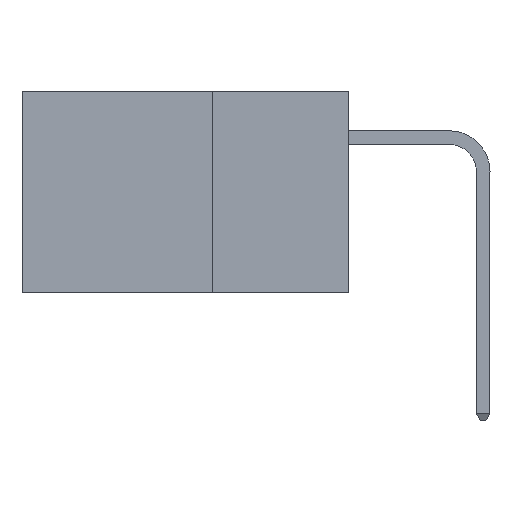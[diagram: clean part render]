
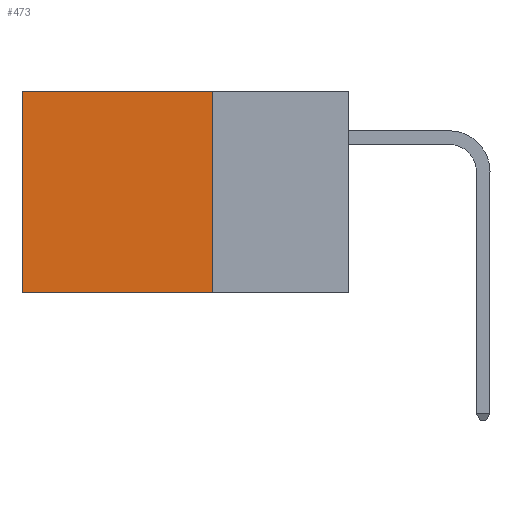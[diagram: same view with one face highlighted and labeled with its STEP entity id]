
A CAD part, left-side view. The second image highlights one B-rep face of the part: STEP entity #473.
In plain terms, the highlighted planar face has unit normal (-1, 0, 0).
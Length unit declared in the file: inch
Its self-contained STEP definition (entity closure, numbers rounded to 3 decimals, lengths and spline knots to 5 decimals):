
#473 = ADVANCED_FACE ( 'NONE', ( #1772 ), #3914, .F. ) ;
#619 = ORIENTED_EDGE ( 'NONE', *, *, #7705, .T. ) ;
#861 = VECTOR ( 'NONE', #3356, 39.37008 ) ;
#919 = EDGE_CURVE ( 'NONE', #1780, #6752, #3969, .T. ) ;
#1046 = VERTEX_POINT ( 'NONE', #3872 ) ;
#1772 = FACE_OUTER_BOUND ( 'NONE', #5500, .T. ) ;
#1780 = VERTEX_POINT ( 'NONE', #4037 ) ;
#1811 = ORIENTED_EDGE ( 'NONE', *, *, #919, .F. ) ;
#2061 = LINE ( 'NONE', #7927, #3996 ) ;
#3240 = LINE ( 'NONE', #6146, #7580 ) ;
#3356 = DIRECTION ( 'NONE',  ( 0., 1., 0. ) ) ;
#3872 = CARTESIAN_POINT ( 'NONE',  ( 0.2875, 0.25, 0. ) ) ;
#3914 = PLANE ( 'NONE',  #4721 ) ;
#3929 = CARTESIAN_POINT ( 'NONE',  ( 0.2875, 0.25, 0. ) ) ;
#3969 = LINE ( 'NONE', #9675, #10217 ) ;
#3996 = VECTOR ( 'NONE', #8744, 39.37008 ) ;
#4037 = CARTESIAN_POINT ( 'NONE',  ( 0.2875, 0.25, -0.37 ) ) ;
#4500 = DIRECTION ( 'NONE',  ( 1., 0., 0. ) ) ;
#4523 = DIRECTION ( 'NONE',  ( 0., 0., -1. ) ) ;
#4721 = AXIS2_PLACEMENT_3D ( 'NONE', #3929, #4500, #4523 ) ;
#4950 = DIRECTION ( 'NONE',  ( 0., 1., 0. ) ) ;
#5408 = CARTESIAN_POINT ( 'NONE',  ( 0.2875, 0.6, 0. ) ) ;
#5500 = EDGE_LOOP ( 'NONE', ( #7811, #1811, #8606, #619 ) ) ;
#5588 = EDGE_CURVE ( 'NONE', #1046, #1780, #3240, .T. ) ;
#6146 = CARTESIAN_POINT ( 'NONE',  ( 0.2875, 0.25, 0. ) ) ;
#6162 = DIRECTION ( 'NONE',  ( 0., 0., -1. ) ) ;
#6752 = VERTEX_POINT ( 'NONE', #10094 ) ;
#6909 = EDGE_CURVE ( 'NONE', #7962, #6752, #2061, .T. ) ;
#7580 = VECTOR ( 'NONE', #6162, 39.37008 ) ;
#7705 = EDGE_CURVE ( 'NONE', #1046, #7962, #8713, .T. ) ;
#7811 = ORIENTED_EDGE ( 'NONE', *, *, #6909, .T. ) ;
#7927 = CARTESIAN_POINT ( 'NONE',  ( 0.2875, 0.6, 0. ) ) ;
#7962 = VERTEX_POINT ( 'NONE', #5408 ) ;
#8316 = CARTESIAN_POINT ( 'NONE',  ( 0.2875, 0.25, 0. ) ) ;
#8606 = ORIENTED_EDGE ( 'NONE', *, *, #5588, .F. ) ;
#8713 = LINE ( 'NONE', #8316, #861 ) ;
#8744 = DIRECTION ( 'NONE',  ( 0., 0., -1. ) ) ;
#9675 = CARTESIAN_POINT ( 'NONE',  ( 0.2875, 0.25, -0.37 ) ) ;
#10094 = CARTESIAN_POINT ( 'NONE',  ( 0.2875, 0.6, -0.37 ) ) ;
#10217 = VECTOR ( 'NONE', #4950, 39.37008 ) ;
